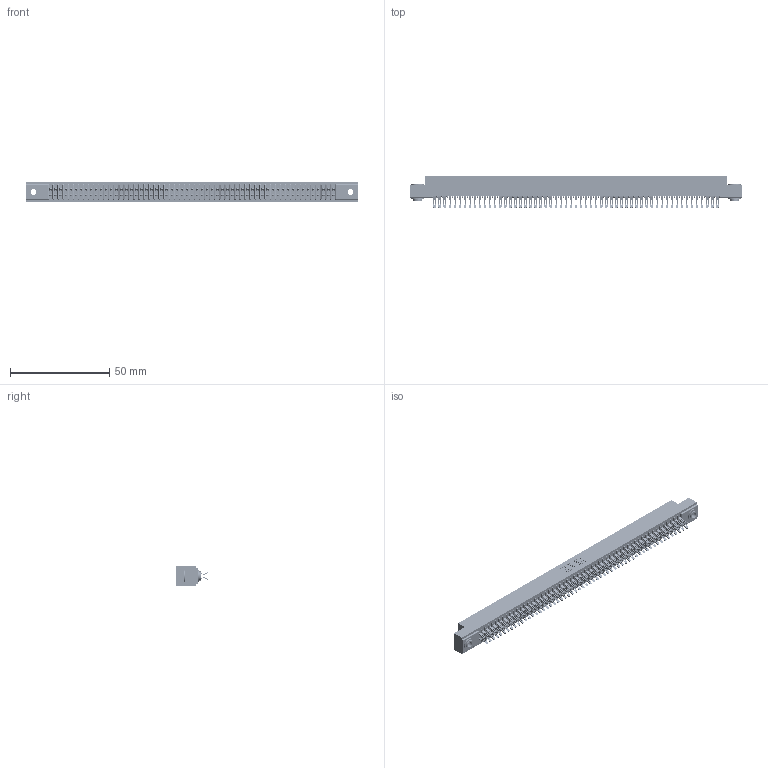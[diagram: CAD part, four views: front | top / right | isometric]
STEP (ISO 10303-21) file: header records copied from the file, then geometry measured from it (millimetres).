
FILE_DESCRIPTION (( 'STEP AP203' ), '1' );
FILE_NAME ('391-114-555-203.STEP', '2018-08-09T22:48:24', ( '' ), ( '' ), 'SwSTEP 2.0', 'SolidWorks 2016', '' );
FILE_SCHEMA (( 'CONFIG_CONTROL_DESIGN' ));
Length unit declared in the file: inch
Products named in the file (4): 341 Part_.156 (3.96) Dia Mounting Holes; 341-292-001_341-292-155; 345-250-002_345-250-002-102; 391-114-555-203
Assembly tree (117 placements, depth 2):
  391-114-555-203
    341 Part_.156 (3.96) Dia Mounting Holes
    341-292-001_341-292-155  x114
    345-250-002_345-250-002-102  x2
Bounding box: 167 x 16.31 x 10.16 mm (x, y, z)
Volume: 12491.9 mm3; surface area: 23822.9 mm2
Topology: 117 solids, 117 shells, 9060 faces, 27047 edges, 17606 vertices
Faces by surface type: plane 4880, cylinder 3944, sphere 116, torus 112, cone 8
Entity records: 68519 total; most frequent: CARTESIAN_POINT 11386, ORIENTED_EDGE 11298, DIRECTION 11045, EDGE_CURVE 5649, VECTOR 4555, LINE 4555, VERTEX_POINT 3570, AXIS2_PLACEMENT_3D 3245
